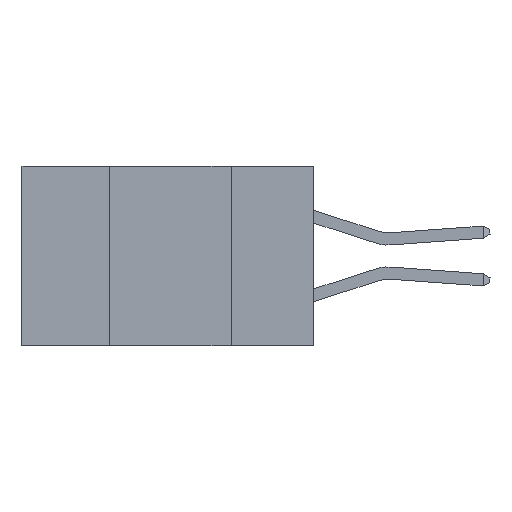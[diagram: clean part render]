
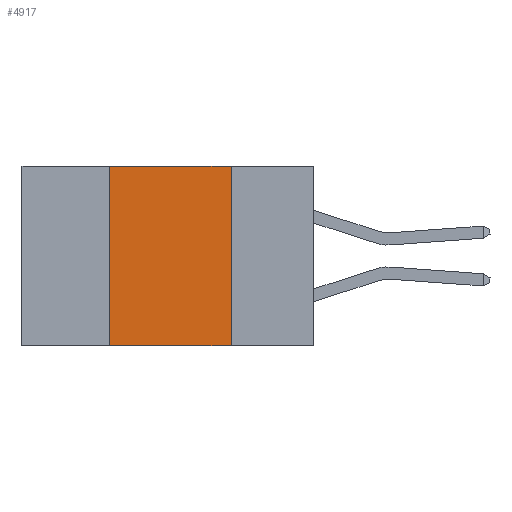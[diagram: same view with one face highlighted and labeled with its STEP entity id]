
A CAD part, left-side view. The second image highlights one B-rep face of the part: STEP entity #4917.
In plain terms, the highlighted planar face has unit normal (-1, 0, 0).
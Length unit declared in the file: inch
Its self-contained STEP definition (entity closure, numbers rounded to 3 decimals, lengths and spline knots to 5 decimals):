
#2548 = DIRECTION ( 'NONE',  ( 0., -1., 0. ) ) ;
#2634 = VERTEX_POINT ( 'NONE', #21159 ) ;
#3500 = DIRECTION ( 'NONE',  ( 1., 0., 0. ) ) ;
#4917 = ADVANCED_FACE ( 'NONE', ( #26156 ), #15651, .F. ) ;
#6333 = EDGE_CURVE ( 'NONE', #13131, #26807, #8469, .T. ) ;
#6665 = EDGE_LOOP ( 'NONE', ( #24976, #33289, #26413, #24622 ) ) ;
#6936 = DIRECTION ( 'NONE',  ( 0., 0., 1. ) ) ;
#7790 = EDGE_CURVE ( 'NONE', #36141, #2634, #16247, .T. ) ;
#8407 = VECTOR ( 'NONE', #30738, 39.37008 ) ;
#8469 = LINE ( 'NONE', #33462, #9384 ) ;
#9384 = VECTOR ( 'NONE', #6936, 39.37008 ) ;
#12802 = CARTESIAN_POINT ( 'NONE',  ( 0., 0.42, 0. ) ) ;
#13131 = VERTEX_POINT ( 'NONE', #29132 ) ;
#13182 = LINE ( 'NONE', #13970, #34016 ) ;
#13970 = CARTESIAN_POINT ( 'NONE',  ( 0., 0.6, -0.37 ) ) ;
#15651 = PLANE ( 'NONE',  #21889 ) ;
#15954 = CARTESIAN_POINT ( 'NONE',  ( 0., 0.17, 0. ) ) ;
#16247 = LINE ( 'NONE', #15954, #8407 ) ;
#18116 = DIRECTION ( 'NONE',  ( 0., 0., -1. ) ) ;
#20013 = CARTESIAN_POINT ( 'NONE',  ( 0., 0.17, 0. ) ) ;
#21159 = CARTESIAN_POINT ( 'NONE',  ( 0., 0.17, -0.37 ) ) ;
#21889 = AXIS2_PLACEMENT_3D ( 'NONE', #24337, #3500, #18116 ) ;
#24337 = CARTESIAN_POINT ( 'NONE',  ( 0., 0.6, 0. ) ) ;
#24622 = ORIENTED_EDGE ( 'NONE', *, *, #31296, .T. ) ;
#24976 = ORIENTED_EDGE ( 'NONE', *, *, #7790, .F. ) ;
#26156 = FACE_OUTER_BOUND ( 'NONE', #6665, .T. ) ;
#26413 = ORIENTED_EDGE ( 'NONE', *, *, #6333, .F. ) ;
#26807 = VERTEX_POINT ( 'NONE', #12802 ) ;
#29132 = CARTESIAN_POINT ( 'NONE',  ( 0., 0.42, -0.37 ) ) ;
#30738 = DIRECTION ( 'NONE',  ( 0., 0., -1. ) ) ;
#31296 = EDGE_CURVE ( 'NONE', #13131, #2634, #13182, .T. ) ;
#31323 = EDGE_CURVE ( 'NONE', #26807, #36141, #35863, .T. ) ;
#33289 = ORIENTED_EDGE ( 'NONE', *, *, #31323, .F. ) ;
#33462 = CARTESIAN_POINT ( 'NONE',  ( 0., 0.42, 0. ) ) ;
#34016 = VECTOR ( 'NONE', #37905, 39.37008 ) ;
#34932 = CARTESIAN_POINT ( 'NONE',  ( 0., 0.6, 0. ) ) ;
#35863 = LINE ( 'NONE', #34932, #36807 ) ;
#36141 = VERTEX_POINT ( 'NONE', #20013 ) ;
#36807 = VECTOR ( 'NONE', #2548, 39.37008 ) ;
#37905 = DIRECTION ( 'NONE',  ( 0., -1., 0. ) ) ;
